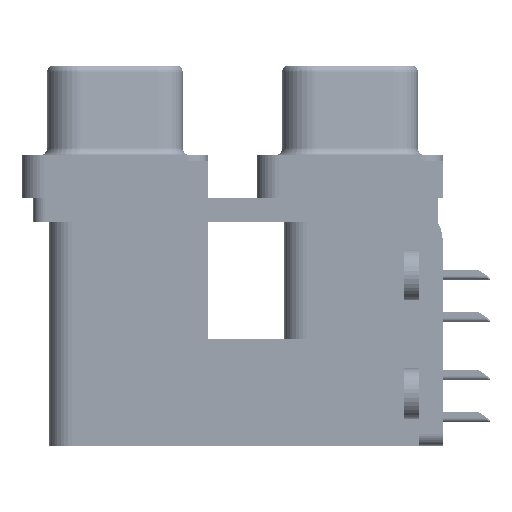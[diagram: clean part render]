
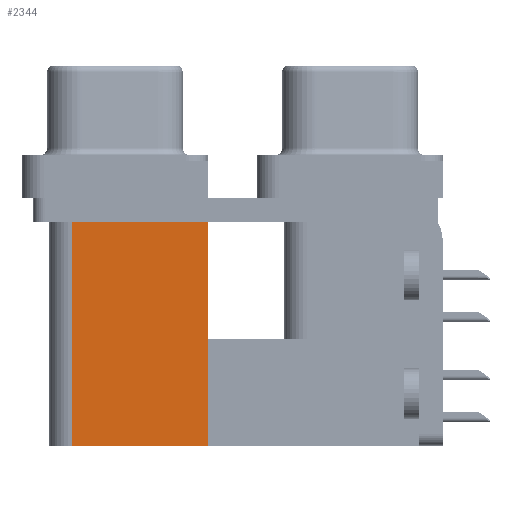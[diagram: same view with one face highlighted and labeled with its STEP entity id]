
A CAD part, left-side view. The second image highlights one B-rep face of the part: STEP entity #2344.
In plain terms, the highlighted planar face has unit normal (-1, 0, 0).
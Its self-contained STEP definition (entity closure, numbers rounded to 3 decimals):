
#827 = CARTESIAN_POINT ( 'NONE',  ( 3.79, 18.8, -2.5 ) ) ;
#2344 = ADVANCED_FACE ( 'NONE', ( #29540 ), #33650, .F. ) ;
#3539 = CARTESIAN_POINT ( 'NONE',  ( 3.79, 9.6, -2.5 ) ) ;
#4079 = VECTOR ( 'NONE', #45913, 1000. ) ;
#8561 = ORIENTED_EDGE ( 'NONE', *, *, #11097, .F. ) ;
#9293 = LINE ( 'NONE', #29368, #10636 ) ;
#9424 = EDGE_CURVE ( 'NONE', #20372, #25571, #9293, .T. ) ;
#10636 = VECTOR ( 'NONE', #10759, 1000. ) ;
#10759 = DIRECTION ( 'NONE',  ( 0., 1., 0. ) ) ;
#10882 = ORIENTED_EDGE ( 'NONE', *, *, #9424, .T. ) ;
#11097 = EDGE_CURVE ( 'NONE', #17194, #25571, #28561, .T. ) ;
#12342 = DIRECTION ( 'NONE',  ( 0., 0., 1. ) ) ;
#17194 = VERTEX_POINT ( 'NONE', #33506 ) ;
#18115 = CARTESIAN_POINT ( 'NONE',  ( 3.79, 9.6, -19.2 ) ) ;
#18966 = CARTESIAN_POINT ( 'NONE',  ( 3.79, 9.6, -19.2 ) ) ;
#20372 = VERTEX_POINT ( 'NONE', #3539 ) ;
#21421 = VECTOR ( 'NONE', #12342, 1000. ) ;
#21466 = DIRECTION ( 'NONE',  ( 0., 1., 0. ) ) ;
#24531 = AXIS2_PLACEMENT_3D ( 'NONE', #18966, #30311, #41393 ) ;
#25571 = VERTEX_POINT ( 'NONE', #827 ) ;
#27071 = VECTOR ( 'NONE', #21466, 1000. ) ;
#28561 = LINE ( 'NONE', #44522, #21421 ) ;
#29194 = LINE ( 'NONE', #18115, #27071 ) ;
#29368 = CARTESIAN_POINT ( 'NONE',  ( 3.79, 9.6, -2.5 ) ) ;
#29540 = FACE_OUTER_BOUND ( 'NONE', #33182, .T. ) ;
#30311 = DIRECTION ( 'NONE',  ( 1., 0., 0. ) ) ;
#33182 = EDGE_LOOP ( 'NONE', ( #10882, #8561, #34918, #49302 ) ) ;
#33506 = CARTESIAN_POINT ( 'NONE',  ( 3.79, 18.8, -19.2 ) ) ;
#33650 = PLANE ( 'NONE',  #24531 ) ;
#34918 = ORIENTED_EDGE ( 'NONE', *, *, #43327, .F. ) ;
#41393 = DIRECTION ( 'NONE',  ( 0., 0., -1. ) ) ;
#42808 = CARTESIAN_POINT ( 'NONE',  ( 3.79, 9.6, -19.2 ) ) ;
#43327 = EDGE_CURVE ( 'NONE', #47536, #17194, #29194, .T. ) ;
#43908 = CARTESIAN_POINT ( 'NONE',  ( 3.79, 9.6, -19.2 ) ) ;
#44522 = CARTESIAN_POINT ( 'NONE',  ( 3.79, 18.8, -19.2 ) ) ;
#45244 = EDGE_CURVE ( 'NONE', #47536, #20372, #50506, .T. ) ;
#45913 = DIRECTION ( 'NONE',  ( 0., 0., 1. ) ) ;
#47536 = VERTEX_POINT ( 'NONE', #43908 ) ;
#49302 = ORIENTED_EDGE ( 'NONE', *, *, #45244, .T. ) ;
#50506 = LINE ( 'NONE', #42808, #4079 ) ;
